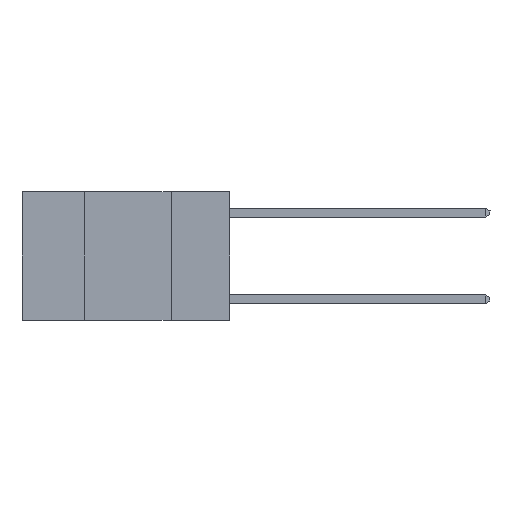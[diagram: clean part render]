
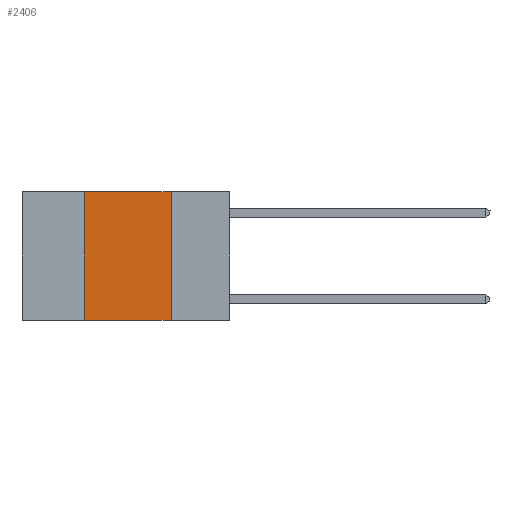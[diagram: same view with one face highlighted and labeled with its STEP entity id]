
A CAD part, left-side view. The second image highlights one B-rep face of the part: STEP entity #2406.
In plain terms, the highlighted planar face has unit normal (-1, 0, 0).
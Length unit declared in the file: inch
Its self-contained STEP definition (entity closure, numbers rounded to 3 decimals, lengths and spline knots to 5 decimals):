
#591 = ORIENTED_EDGE ( 'NONE', *, *, #2305, .F. ) ;
#951 = EDGE_LOOP ( 'NONE', ( #591, #1561, #5720, #1049 ) ) ;
#1008 = AXIS2_PLACEMENT_3D ( 'NONE', #7790, #8560, #3867 ) ;
#1049 = ORIENTED_EDGE ( 'NONE', *, *, #1279, .T. ) ;
#1279 = EDGE_CURVE ( 'NONE', #1462, #7180, #6342, .T. ) ;
#1283 = CARTESIAN_POINT ( 'NONE',  ( 0., 0.17, -0.37 ) ) ;
#1462 = VERTEX_POINT ( 'NONE', #9574 ) ;
#1561 = ORIENTED_EDGE ( 'NONE', *, *, #5684, .F. ) ;
#2284 = PLANE ( 'NONE',  #1008 ) ;
#2305 = EDGE_CURVE ( 'NONE', #6069, #7180, #3857, .T. ) ;
#2406 = ADVANCED_FACE ( 'NONE', ( #4218 ), #2284, .F. ) ;
#2989 = CARTESIAN_POINT ( 'NONE',  ( 0., 0.6, 0. ) ) ;
#3042 = CARTESIAN_POINT ( 'NONE',  ( 0., 0.6, -0.37 ) ) ;
#3148 = CARTESIAN_POINT ( 'NONE',  ( 0., 0.42, 0. ) ) ;
#3663 = CARTESIAN_POINT ( 'NONE',  ( 0., 0.42, 0. ) ) ;
#3857 = LINE ( 'NONE', #8390, #9554 ) ;
#3867 = DIRECTION ( 'NONE',  ( 0., 0., -1. ) ) ;
#4218 = FACE_OUTER_BOUND ( 'NONE', #951, .T. ) ;
#4435 = DIRECTION ( 'NONE',  ( 0., 0., 1. ) ) ;
#4618 = LINE ( 'NONE', #3663, #8308 ) ;
#4786 = VERTEX_POINT ( 'NONE', #3148 ) ;
#5153 = LINE ( 'NONE', #2989, #9508 ) ;
#5684 = EDGE_CURVE ( 'NONE', #4786, #6069, #5153, .T. ) ;
#5720 = ORIENTED_EDGE ( 'NONE', *, *, #8661, .F. ) ;
#6069 = VERTEX_POINT ( 'NONE', #9376 ) ;
#6342 = LINE ( 'NONE', #3042, #7944 ) ;
#7180 = VERTEX_POINT ( 'NONE', #1283 ) ;
#7790 = CARTESIAN_POINT ( 'NONE',  ( 0., 0.6, 0. ) ) ;
#7944 = VECTOR ( 'NONE', #9986, 39.37008 ) ;
#8308 = VECTOR ( 'NONE', #4435, 39.37008 ) ;
#8390 = CARTESIAN_POINT ( 'NONE',  ( 0., 0.17, 0. ) ) ;
#8455 = DIRECTION ( 'NONE',  ( 0., -1., 0. ) ) ;
#8560 = DIRECTION ( 'NONE',  ( 1., 0., 0. ) ) ;
#8661 = EDGE_CURVE ( 'NONE', #1462, #4786, #4618, .T. ) ;
#9145 = DIRECTION ( 'NONE',  ( 0., 0., -1. ) ) ;
#9376 = CARTESIAN_POINT ( 'NONE',  ( 0., 0.17, 0. ) ) ;
#9508 = VECTOR ( 'NONE', #8455, 39.37008 ) ;
#9554 = VECTOR ( 'NONE', #9145, 39.37008 ) ;
#9574 = CARTESIAN_POINT ( 'NONE',  ( 0., 0.42, -0.37 ) ) ;
#9986 = DIRECTION ( 'NONE',  ( 0., -1., 0. ) ) ;
